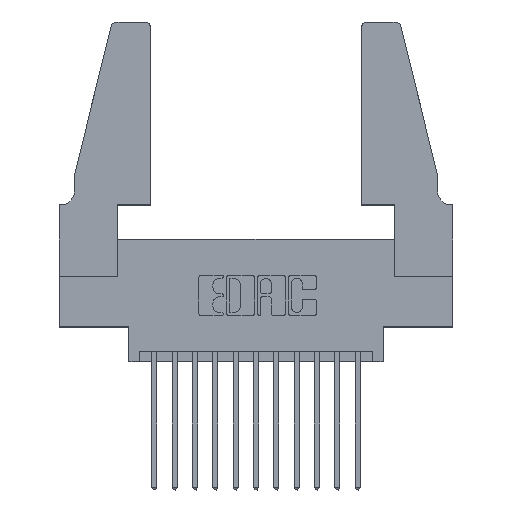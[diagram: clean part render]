
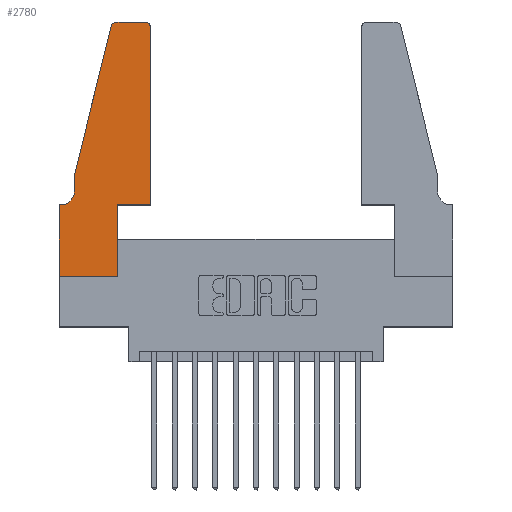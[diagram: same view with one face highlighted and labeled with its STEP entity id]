
A CAD part, top view. The second image highlights one B-rep face of the part: STEP entity #2780.
In plain terms, the highlighted planar face has unit normal (0, 0, 1).
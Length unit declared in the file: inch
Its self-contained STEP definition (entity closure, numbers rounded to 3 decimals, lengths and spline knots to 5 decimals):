
#47 = ORIENTED_EDGE ( 'NONE', *, *, #8459, .T. ) ;
#48 = VECTOR ( 'NONE', #5341, 39.37008 ) ;
#77 = ORIENTED_EDGE ( 'NONE', *, *, #11273, .T. ) ;
#126 = VERTEX_POINT ( 'NONE', #8757 ) ;
#129 = CARTESIAN_POINT ( 'NONE',  ( 0.4505, 0.35, 0.37 ) ) ;
#311 = VERTEX_POINT ( 'NONE', #10711 ) ;
#340 = EDGE_CURVE ( 'NONE', #6072, #7725, #12271, .T. ) ;
#465 = CARTESIAN_POINT ( 'NONE',  ( 0.2865, 0.35, 0.37 ) ) ;
#525 = ORIENTED_EDGE ( 'NONE', *, *, #340, .T. ) ;
#615 = DIRECTION ( 'NONE',  ( 0., 0., 1. ) ) ;
#1006 = DIRECTION ( 'NONE',  ( 0., -1., 0. ) ) ;
#1262 = VECTOR ( 'NONE', #1006, 39.37008 ) ;
#1409 = CARTESIAN_POINT ( 'NONE',  ( 0.4205, 1.22, 0.37 ) ) ;
#1410 = CARTESIAN_POINT ( 'NONE',  ( 0., 0.35, 0.37 ) ) ;
#1467 = LINE ( 'NONE', #11889, #9655 ) ;
#1510 = CIRCLE ( 'NONE', #5747, 0.03 ) ;
#1574 = CARTESIAN_POINT ( 'NONE',  ( 0.4505, 0.35, 0.37 ) ) ;
#1662 = VERTEX_POINT ( 'NONE', #2702 ) ;
#1670 = ORIENTED_EDGE ( 'NONE', *, *, #2531, .T. ) ;
#1764 = AXIS2_PLACEMENT_3D ( 'NONE', #1409, #9543, #2657 ) ;
#2531 = EDGE_CURVE ( 'NONE', #11095, #8685, #11604, .T. ) ;
#2657 = DIRECTION ( 'NONE',  ( 1., 0., 0. ) ) ;
#2702 = CARTESIAN_POINT ( 'NONE',  ( 0.2865, 0., 0.37 ) ) ;
#2731 = DIRECTION ( 'NONE',  ( -0.239, -0.971, 0. ) ) ;
#2780 = ADVANCED_FACE ( 'NONE', ( #11053 ), #10720, .T. ) ;
#3386 = EDGE_CURVE ( 'NONE', #9199, #15035, #12293, .T. ) ;
#3416 = CARTESIAN_POINT ( 'NONE',  ( 0., 0., 0.37 ) ) ;
#3833 = VERTEX_POINT ( 'NONE', #465 ) ;
#3845 = DIRECTION ( 'NONE',  ( -1., 0., 0. ) ) ;
#4224 = DIRECTION ( 'NONE',  ( 0., 1., 0. ) ) ;
#4258 = CARTESIAN_POINT ( 'NONE',  ( 0.4505, 1.22, 0.37 ) ) ;
#4291 = VECTOR ( 'NONE', #8361, 39.37008 ) ;
#4759 = AXIS2_PLACEMENT_3D ( 'NONE', #1410, #615, #8220 ) ;
#4818 = LINE ( 'NONE', #3416, #1262 ) ;
#4868 = DIRECTION ( 'NONE',  ( 0., 0., -1. ) ) ;
#5334 = ORIENTED_EDGE ( 'NONE', *, *, #8421, .T. ) ;
#5341 = DIRECTION ( 'NONE',  ( 1., 0., 0. ) ) ;
#5415 = DIRECTION ( 'NONE',  ( 0., 1., 0. ) ) ;
#5592 = DIRECTION ( 'NONE',  ( 0., -1., 0. ) ) ;
#5747 = AXIS2_PLACEMENT_3D ( 'NONE', #5952, #14005, #7097 ) ;
#5952 = CARTESIAN_POINT ( 'NONE',  ( 0.284, 1.22, 0.37 ) ) ;
#6072 = VERTEX_POINT ( 'NONE', #10501 ) ;
#6845 = VERTEX_POINT ( 'NONE', #11128 ) ;
#6898 = ORIENTED_EDGE ( 'NONE', *, *, #7597, .T. ) ;
#7097 = DIRECTION ( 'NONE',  ( 1., 0., 0. ) ) ;
#7445 = CARTESIAN_POINT ( 'NONE',  ( 0.0755, 0.5, 0.37 ) ) ;
#7597 = EDGE_CURVE ( 'NONE', #311, #6845, #4818, .T. ) ;
#7687 = VECTOR ( 'NONE', #2731, 39.37008 ) ;
#7725 = VERTEX_POINT ( 'NONE', #14048 ) ;
#7843 = EDGE_CURVE ( 'NONE', #9208, #9199, #13446, .T. ) ;
#8180 = VECTOR ( 'NONE', #4224, 39.37008 ) ;
#8220 = DIRECTION ( 'NONE',  ( 1., 0., 0. ) ) ;
#8345 = VECTOR ( 'NONE', #5415, 39.37008 ) ;
#8361 = DIRECTION ( 'NONE',  ( 1., 0., 0. ) ) ;
#8421 = EDGE_CURVE ( 'NONE', #3833, #11095, #13465, .T. ) ;
#8459 = EDGE_CURVE ( 'NONE', #126, #311, #1467, .T. ) ;
#8476 = VECTOR ( 'NONE', #10202, 39.37008 ) ;
#8636 = EDGE_LOOP ( 'NONE', ( #525, #8769, #13735, #10048, #10106, #47, #6898, #13777, #77, #5334, #1670, #9629 ) ) ;
#8685 = VERTEX_POINT ( 'NONE', #4258 ) ;
#8757 = CARTESIAN_POINT ( 'NONE',  ( 0.0055, 0.35, 0.37 ) ) ;
#8769 = ORIENTED_EDGE ( 'NONE', *, *, #13794, .T. ) ;
#9199 = VERTEX_POINT ( 'NONE', #7445 ) ;
#9208 = VERTEX_POINT ( 'NONE', #12069 ) ;
#9214 = CIRCLE ( 'NONE', #1764, 0.03 ) ;
#9543 = DIRECTION ( 'NONE',  ( 0., 0., 1. ) ) ;
#9614 = CARTESIAN_POINT ( 'NONE',  ( 0.0755, 0.5, 0.37 ) ) ;
#9629 = ORIENTED_EDGE ( 'NONE', *, *, #11008, .T. ) ;
#9655 = VECTOR ( 'NONE', #3845, 39.37008 ) ;
#10048 = ORIENTED_EDGE ( 'NONE', *, *, #3386, .T. ) ;
#10056 = EDGE_CURVE ( 'NONE', #6845, #1662, #12496, .T. ) ;
#10106 = ORIENTED_EDGE ( 'NONE', *, *, #14484, .T. ) ;
#10155 = CARTESIAN_POINT ( 'NONE',  ( 0.2605, 1.25, 0.37 ) ) ;
#10202 = DIRECTION ( 'NONE',  ( -1., 0., 0. ) ) ;
#10501 = CARTESIAN_POINT ( 'NONE',  ( 0.4205, 1.25, 0.37 ) ) ;
#10711 = CARTESIAN_POINT ( 'NONE',  ( 0., 0.35, 0.37 ) ) ;
#10720 = PLANE ( 'NONE',  #4759 ) ;
#11008 = EDGE_CURVE ( 'NONE', #8685, #6072, #9214, .T. ) ;
#11053 = FACE_OUTER_BOUND ( 'NONE', #8636, .T. ) ;
#11095 = VERTEX_POINT ( 'NONE', #1574 ) ;
#11128 = CARTESIAN_POINT ( 'NONE',  ( 0., 0., 0.37 ) ) ;
#11273 = EDGE_CURVE ( 'NONE', #1662, #3833, #11412, .T. ) ;
#11412 = LINE ( 'NONE', #13448, #8345 ) ;
#11580 = CARTESIAN_POINT ( 'NONE',  ( 0.0755, 0.42, 0.37 ) ) ;
#11604 = LINE ( 'NONE', #129, #8180 ) ;
#11748 = CARTESIAN_POINT ( 'NONE',  ( 0.0055, 0.42, 0.37 ) ) ;
#11889 = CARTESIAN_POINT ( 'NONE',  ( 0.0755, 0.35, 0.37 ) ) ;
#11933 = VECTOR ( 'NONE', #5592, 39.37008 ) ;
#12069 = CARTESIAN_POINT ( 'NONE',  ( 0.25487, 1.22718, 0.37 ) ) ;
#12216 = CARTESIAN_POINT ( 'NONE',  ( 0., 0., 0.37 ) ) ;
#12271 = LINE ( 'NONE', #10155, #8476 ) ;
#12293 = LINE ( 'NONE', #15031, #11933 ) ;
#12496 = LINE ( 'NONE', #12216, #48 ) ;
#12909 = DIRECTION ( 'NONE',  ( -1., 0., 0. ) ) ;
#13446 = LINE ( 'NONE', #9614, #7687 ) ;
#13448 = CARTESIAN_POINT ( 'NONE',  ( 0.2865, 0.35, 0.37 ) ) ;
#13465 = LINE ( 'NONE', #14124, #4291 ) ;
#13735 = ORIENTED_EDGE ( 'NONE', *, *, #7843, .T. ) ;
#13777 = ORIENTED_EDGE ( 'NONE', *, *, #10056, .T. ) ;
#13794 = EDGE_CURVE ( 'NONE', #7725, #9208, #1510, .T. ) ;
#14005 = DIRECTION ( 'NONE',  ( 0., 0., 1. ) ) ;
#14048 = CARTESIAN_POINT ( 'NONE',  ( 0.284, 1.25, 0.37 ) ) ;
#14124 = CARTESIAN_POINT ( 'NONE',  ( 0.4505, 0.35, 0.37 ) ) ;
#14426 = AXIS2_PLACEMENT_3D ( 'NONE', #11748, #4868, #12909 ) ;
#14454 = CIRCLE ( 'NONE', #14426, 0.07 ) ;
#14484 = EDGE_CURVE ( 'NONE', #15035, #126, #14454, .T. ) ;
#15031 = CARTESIAN_POINT ( 'NONE',  ( 0.0755, 0.5, 0.37 ) ) ;
#15035 = VERTEX_POINT ( 'NONE', #11580 ) ;
